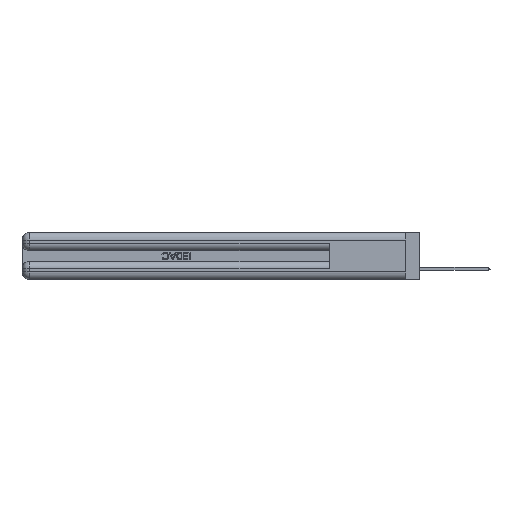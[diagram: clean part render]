
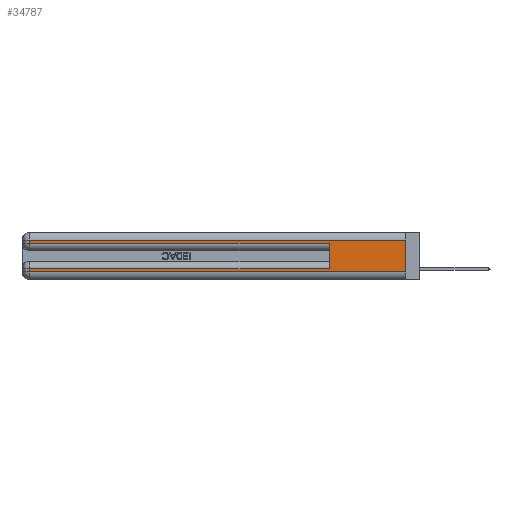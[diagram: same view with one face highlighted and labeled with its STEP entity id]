
A CAD part, left-side view. The second image highlights one B-rep face of the part: STEP entity #34787.
In plain terms, the highlighted planar face has unit normal (-1, 0, 0).
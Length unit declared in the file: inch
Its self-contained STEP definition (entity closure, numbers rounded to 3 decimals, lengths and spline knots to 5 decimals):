
#88 = EDGE_CURVE ( 'NONE', #13980, #22720, #4731, .T. ) ;
#999 = FACE_OUTER_BOUND ( 'NONE', #11098, .T. ) ;
#1486 = CARTESIAN_POINT ( 'NONE',  ( 0., 0., 0.31 ) ) ;
#1745 = CARTESIAN_POINT ( 'NONE',  ( 0., 2.94, 0.31 ) ) ;
#1992 = DIRECTION ( 'NONE',  ( 0., -1., 0. ) ) ;
#2456 = EDGE_CURVE ( 'NONE', #23060, #13980, #12273, .T. ) ;
#3541 = CARTESIAN_POINT ( 'NONE',  ( 0., 0., 0.085 ) ) ;
#4209 = VECTOR ( 'NONE', #37165, 39.37008 ) ;
#4594 = EDGE_CURVE ( 'NONE', #5239, #15239, #32104, .T. ) ;
#4731 = LINE ( 'NONE', #48483, #17275 ) ;
#4761 = ORIENTED_EDGE ( 'NONE', *, *, #40330, .T. ) ;
#4917 = ORIENTED_EDGE ( 'NONE', *, *, #4594, .T. ) ;
#4930 = VECTOR ( 'NONE', #15410, 39.37008 ) ;
#5111 = VERTEX_POINT ( 'NONE', #25633 ) ;
#5239 = VERTEX_POINT ( 'NONE', #1745 ) ;
#6077 = DIRECTION ( 'NONE',  ( 0., 0., -1. ) ) ;
#6969 = ORIENTED_EDGE ( 'NONE', *, *, #27809, .T. ) ;
#7043 = CARTESIAN_POINT ( 'NONE',  ( 0., 2.94, 0.06 ) ) ;
#7353 = ORIENTED_EDGE ( 'NONE', *, *, #2456, .T. ) ;
#7894 = LINE ( 'NONE', #11147, #4930 ) ;
#9810 = CARTESIAN_POINT ( 'NONE',  ( 0., 0., 0.285 ) ) ;
#11098 = EDGE_LOOP ( 'NONE', ( #43017, #30082, #4917, #4761, #39141, #7353, #38217, #6969 ) ) ;
#11147 = CARTESIAN_POINT ( 'NONE',  ( 0., 0., 0.37 ) ) ;
#12273 = LINE ( 'NONE', #3541, #20699 ) ;
#12372 = VECTOR ( 'NONE', #1992, 39.37008 ) ;
#13980 = VERTEX_POINT ( 'NONE', #36197 ) ;
#14198 = DIRECTION ( 'NONE',  ( 0., 0., -1. ) ) ;
#14829 = EDGE_CURVE ( 'NONE', #30758, #34486, #7894, .T. ) ;
#15239 = VERTEX_POINT ( 'NONE', #20797 ) ;
#15410 = DIRECTION ( 'NONE',  ( 0., 0., -1. ) ) ;
#17164 = DIRECTION ( 'NONE',  ( 1., 0., 0. ) ) ;
#17275 = VECTOR ( 'NONE', #14198, 39.37008 ) ;
#19139 = LINE ( 'NONE', #26802, #31601 ) ;
#20699 = VECTOR ( 'NONE', #26482, 39.37008 ) ;
#20797 = CARTESIAN_POINT ( 'NONE',  ( 0., 2.94, 0.285 ) ) ;
#22610 = VECTOR ( 'NONE', #6077, 39.37008 ) ;
#22720 = VERTEX_POINT ( 'NONE', #7043 ) ;
#23060 = VERTEX_POINT ( 'NONE', #48023 ) ;
#24908 = LINE ( 'NONE', #9810, #12372 ) ;
#25633 = CARTESIAN_POINT ( 'NONE',  ( 0., 0.6, 0.285 ) ) ;
#26482 = DIRECTION ( 'NONE',  ( 0., 1., 0. ) ) ;
#26802 = CARTESIAN_POINT ( 'NONE',  ( 0., 0.6, 0.145 ) ) ;
#27809 = EDGE_CURVE ( 'NONE', #22720, #34486, #37030, .T. ) ;
#30082 = ORIENTED_EDGE ( 'NONE', *, *, #46174, .T. ) ;
#30758 = VERTEX_POINT ( 'NONE', #31010 ) ;
#31010 = CARTESIAN_POINT ( 'NONE',  ( 0., 0., 0.31 ) ) ;
#31601 = VECTOR ( 'NONE', #34651, 39.37008 ) ;
#32104 = LINE ( 'NONE', #35135, #22610 ) ;
#33221 = EDGE_CURVE ( 'NONE', #23060, #5111, #19139, .T. ) ;
#33476 = CARTESIAN_POINT ( 'NONE',  ( 0., 0., 0.06 ) ) ;
#33523 = CARTESIAN_POINT ( 'NONE',  ( 0., 0., 0.06 ) ) ;
#34486 = VERTEX_POINT ( 'NONE', #33523 ) ;
#34651 = DIRECTION ( 'NONE',  ( 0., 0., 1. ) ) ;
#34787 = ADVANCED_FACE ( 'NONE', ( #999 ), #40298, .F. ) ;
#35135 = CARTESIAN_POINT ( 'NONE',  ( 0., 2.94, 0.37 ) ) ;
#35227 = AXIS2_PLACEMENT_3D ( 'NONE', #48273, #17164, #47949 ) ;
#36197 = CARTESIAN_POINT ( 'NONE',  ( 0., 2.94, 0.085 ) ) ;
#36798 = LINE ( 'NONE', #1486, #37451 ) ;
#37030 = LINE ( 'NONE', #33476, #4209 ) ;
#37165 = DIRECTION ( 'NONE',  ( 0., -1., 0. ) ) ;
#37451 = VECTOR ( 'NONE', #47075, 39.37008 ) ;
#38217 = ORIENTED_EDGE ( 'NONE', *, *, #88, .T. ) ;
#39141 = ORIENTED_EDGE ( 'NONE', *, *, #33221, .F. ) ;
#40298 = PLANE ( 'NONE',  #35227 ) ;
#40330 = EDGE_CURVE ( 'NONE', #15239, #5111, #24908, .T. ) ;
#43017 = ORIENTED_EDGE ( 'NONE', *, *, #14829, .F. ) ;
#46174 = EDGE_CURVE ( 'NONE', #30758, #5239, #36798, .T. ) ;
#47075 = DIRECTION ( 'NONE',  ( 0., 1., 0. ) ) ;
#47949 = DIRECTION ( 'NONE',  ( 0., 0., -1. ) ) ;
#48023 = CARTESIAN_POINT ( 'NONE',  ( 0., 0.6, 0.085 ) ) ;
#48273 = CARTESIAN_POINT ( 'NONE',  ( 0., 0., 0.37 ) ) ;
#48483 = CARTESIAN_POINT ( 'NONE',  ( 0., 2.94, 0.37 ) ) ;
